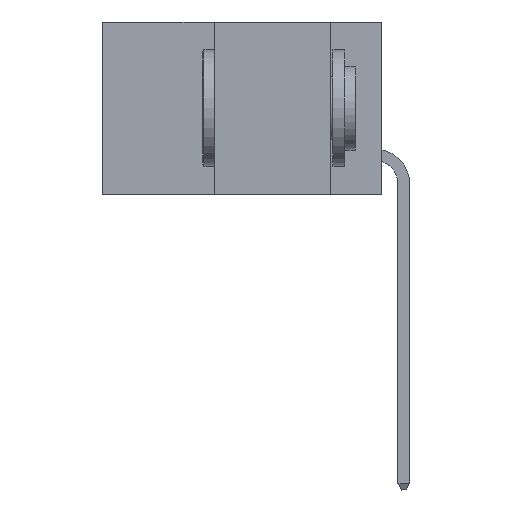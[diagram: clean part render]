
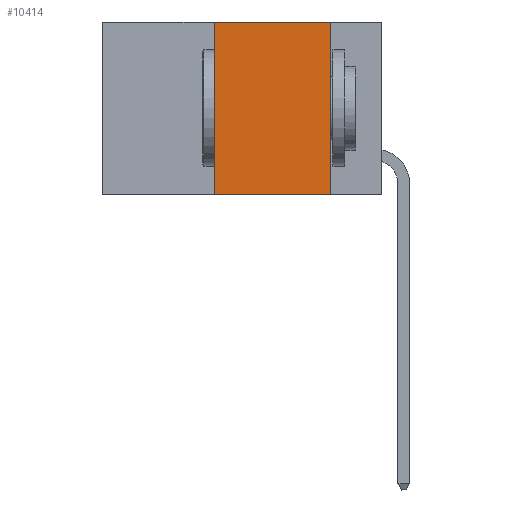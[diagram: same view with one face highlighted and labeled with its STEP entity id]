
A CAD part, left-side view. The second image highlights one B-rep face of the part: STEP entity #10414.
In plain terms, the highlighted planar face has unit normal (-1, 0, 0).
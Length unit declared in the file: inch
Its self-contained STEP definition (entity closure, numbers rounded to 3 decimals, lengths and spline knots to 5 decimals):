
#1546 = VERTEX_POINT ( 'NONE', #19555 ) ;
#2247 = CARTESIAN_POINT ( 'NONE',  ( 0., 0.11, 0. ) ) ;
#2270 = ORIENTED_EDGE ( 'NONE', *, *, #12250, .F. ) ;
#2307 = DIRECTION ( 'NONE',  ( 1., 0., 0. ) ) ;
#3772 = VECTOR ( 'NONE', #16806, 39.37008 ) ;
#4820 = AXIS2_PLACEMENT_3D ( 'NONE', #21905, #2307, #14811 ) ;
#4989 = CARTESIAN_POINT ( 'NONE',  ( 0., 0.6, -0.37 ) ) ;
#5535 = CARTESIAN_POINT ( 'NONE',  ( 0., 0.6, 0. ) ) ;
#5757 = EDGE_LOOP ( 'NONE', ( #11971, #2270, #17391, #16082 ) ) ;
#6537 = LINE ( 'NONE', #5535, #11868 ) ;
#6841 = CARTESIAN_POINT ( 'NONE',  ( 0., 0.11, -0.37 ) ) ;
#8042 = CARTESIAN_POINT ( 'NONE',  ( 0., 0.36, 0. ) ) ;
#8868 = EDGE_CURVE ( 'NONE', #21718, #17125, #14807, .T. ) ;
#9340 = CARTESIAN_POINT ( 'NONE',  ( 0., 0.36, 0. ) ) ;
#10044 = VECTOR ( 'NONE', #11938, 39.37008 ) ;
#10414 = ADVANCED_FACE ( 'NONE', ( #17489 ), #16716, .F. ) ;
#11868 = VECTOR ( 'NONE', #19882, 39.37008 ) ;
#11938 = DIRECTION ( 'NONE',  ( 0., -1., 0. ) ) ;
#11971 = ORIENTED_EDGE ( 'NONE', *, *, #21388, .F. ) ;
#12250 = EDGE_CURVE ( 'NONE', #20733, #1546, #6537, .T. ) ;
#12491 = LINE ( 'NONE', #2247, #3772 ) ;
#13946 = LINE ( 'NONE', #9340, #20113 ) ;
#13972 = EDGE_CURVE ( 'NONE', #21718, #20733, #13946, .T. ) ;
#14807 = LINE ( 'NONE', #4989, #10044 ) ;
#14811 = DIRECTION ( 'NONE',  ( 0., 0., -1. ) ) ;
#16082 = ORIENTED_EDGE ( 'NONE', *, *, #8868, .T. ) ;
#16716 = PLANE ( 'NONE',  #4820 ) ;
#16806 = DIRECTION ( 'NONE',  ( 0., 0., -1. ) ) ;
#17125 = VERTEX_POINT ( 'NONE', #6841 ) ;
#17391 = ORIENTED_EDGE ( 'NONE', *, *, #13972, .F. ) ;
#17489 = FACE_OUTER_BOUND ( 'NONE', #5757, .T. ) ;
#19555 = CARTESIAN_POINT ( 'NONE',  ( 0., 0.11, 0. ) ) ;
#19882 = DIRECTION ( 'NONE',  ( 0., -1., 0. ) ) ;
#20113 = VECTOR ( 'NONE', #21843, 39.37008 ) ;
#20733 = VERTEX_POINT ( 'NONE', #8042 ) ;
#21388 = EDGE_CURVE ( 'NONE', #1546, #17125, #12491, .T. ) ;
#21510 = CARTESIAN_POINT ( 'NONE',  ( 0., 0.36, -0.37 ) ) ;
#21718 = VERTEX_POINT ( 'NONE', #21510 ) ;
#21843 = DIRECTION ( 'NONE',  ( 0., 0., 1. ) ) ;
#21905 = CARTESIAN_POINT ( 'NONE',  ( 0., 0.6, 0. ) ) ;
